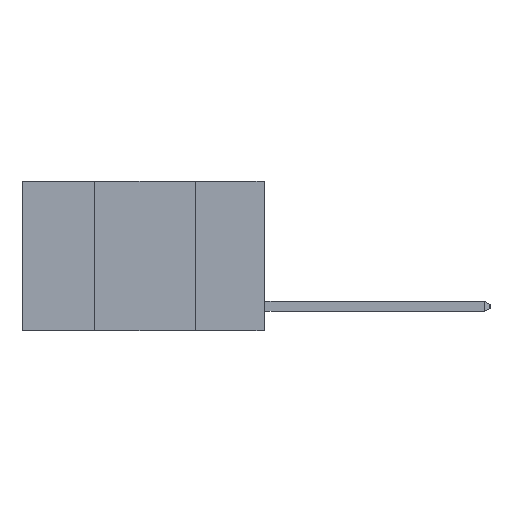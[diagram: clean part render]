
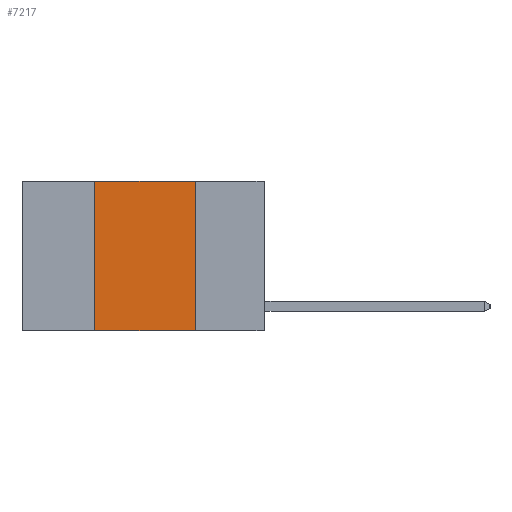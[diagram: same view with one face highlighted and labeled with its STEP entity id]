
A CAD part, left-side view. The second image highlights one B-rep face of the part: STEP entity #7217.
In plain terms, the highlighted planar face has unit normal (-1, 0, 0).
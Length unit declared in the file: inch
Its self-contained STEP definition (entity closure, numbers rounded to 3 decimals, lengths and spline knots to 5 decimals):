
#249 = VERTEX_POINT ( 'NONE', #8993 ) ;
#449 = AXIS2_PLACEMENT_3D ( 'NONE', #2304, #3099, #8710 ) ;
#653 = ORIENTED_EDGE ( 'NONE', *, *, #8158, .T. ) ;
#1075 = CARTESIAN_POINT ( 'NONE',  ( 0., 0.6, -0.37 ) ) ;
#1428 = DIRECTION ( 'NONE',  ( 0., 0., -1. ) ) ;
#1483 = LINE ( 'NONE', #7041, #7390 ) ;
#1994 = FACE_OUTER_BOUND ( 'NONE', #5142, .T. ) ;
#2304 = CARTESIAN_POINT ( 'NONE',  ( 0., 0.6, 0. ) ) ;
#2504 = EDGE_CURVE ( 'NONE', #249, #4248, #10337, .T. ) ;
#3099 = DIRECTION ( 'NONE',  ( 1., 0., 0. ) ) ;
#3325 = CARTESIAN_POINT ( 'NONE',  ( 0., 0.42, 0. ) ) ;
#3405 = VECTOR ( 'NONE', #6718, 39.37008 ) ;
#3510 = ORIENTED_EDGE ( 'NONE', *, *, #2504, .F. ) ;
#4041 = LINE ( 'NONE', #6999, #8070 ) ;
#4248 = VERTEX_POINT ( 'NONE', #5657 ) ;
#4612 = ORIENTED_EDGE ( 'NONE', *, *, #10154, .F. ) ;
#5142 = EDGE_LOOP ( 'NONE', ( #3510, #4612, #9811, #653 ) ) ;
#5275 = LINE ( 'NONE', #1075, #3405 ) ;
#5300 = EDGE_CURVE ( 'NONE', #5727, #6085, #4041, .T. ) ;
#5421 = CARTESIAN_POINT ( 'NONE',  ( 0., 0.17, 0. ) ) ;
#5657 = CARTESIAN_POINT ( 'NONE',  ( 0., 0.17, -0.37 ) ) ;
#5727 = VERTEX_POINT ( 'NONE', #6917 ) ;
#6085 = VERTEX_POINT ( 'NONE', #3325 ) ;
#6718 = DIRECTION ( 'NONE',  ( 0., -1., 0. ) ) ;
#6917 = CARTESIAN_POINT ( 'NONE',  ( 0., 0.42, -0.37 ) ) ;
#6999 = CARTESIAN_POINT ( 'NONE',  ( 0., 0.42, 0. ) ) ;
#7041 = CARTESIAN_POINT ( 'NONE',  ( 0., 0.6, 0. ) ) ;
#7112 = PLANE ( 'NONE',  #449 ) ;
#7217 = ADVANCED_FACE ( 'NONE', ( #1994 ), #7112, .F. ) ;
#7390 = VECTOR ( 'NONE', #9430, 39.37008 ) ;
#8070 = VECTOR ( 'NONE', #10191, 39.37008 ) ;
#8158 = EDGE_CURVE ( 'NONE', #5727, #4248, #5275, .T. ) ;
#8240 = VECTOR ( 'NONE', #1428, 39.37008 ) ;
#8710 = DIRECTION ( 'NONE',  ( 0., 0., -1. ) ) ;
#8993 = CARTESIAN_POINT ( 'NONE',  ( 0., 0.17, 0. ) ) ;
#9430 = DIRECTION ( 'NONE',  ( 0., -1., 0. ) ) ;
#9811 = ORIENTED_EDGE ( 'NONE', *, *, #5300, .F. ) ;
#10154 = EDGE_CURVE ( 'NONE', #6085, #249, #1483, .T. ) ;
#10191 = DIRECTION ( 'NONE',  ( 0., 0., 1. ) ) ;
#10337 = LINE ( 'NONE', #5421, #8240 ) ;
